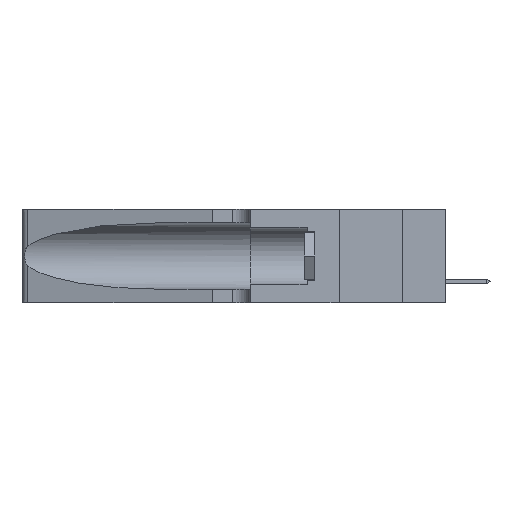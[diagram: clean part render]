
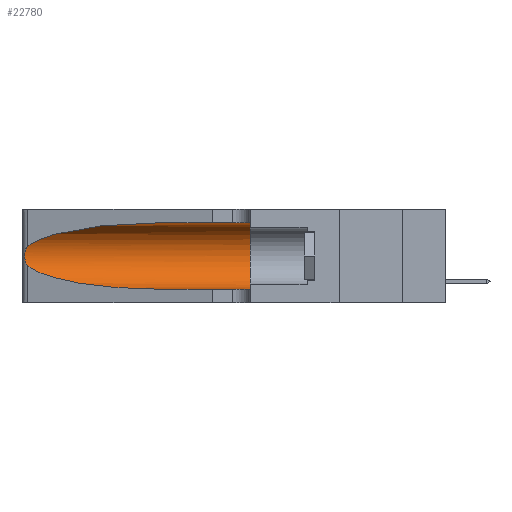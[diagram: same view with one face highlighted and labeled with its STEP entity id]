
A CAD part, left-side view. The second image highlights one B-rep face of the part: STEP entity #22780.
In plain terms, the highlighted cylindrical face has radius 3.308 mm (diameter 6.617 mm), a partial arc.
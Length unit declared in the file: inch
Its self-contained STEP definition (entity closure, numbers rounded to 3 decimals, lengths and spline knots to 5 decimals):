
#247 = ORIENTED_EDGE ( 'NONE', *, *, #14036, .T. ) ;
#489 = EDGE_CURVE ( 'NONE', #13687, #13016, #5493, .T. ) ;
#1385 = CARTESIAN_POINT ( 'NONE',  ( 0.1305, 0.72297, 0.31525 ) ) ;
#1885 = LINE ( 'NONE', #21795, #19134 ) ;
#2237 = CARTESIAN_POINT ( 'NONE',  ( 0.25555, 1.22993, 0.14849 ) ) ;
#2495 = DIRECTION ( 'NONE',  ( 0., -1., 0. ) ) ;
#2584 = CARTESIAN_POINT ( 'NONE',  ( 0.25856, 1.23593, 0.16098 ) ) ;
#2806 = ORIENTED_EDGE ( 'NONE', *, *, #20119, .T. ) ;
#3103 = EDGE_CURVE ( 'NONE', #4375, #17289, #7499, .T. ) ;
#3889 = CARTESIAN_POINT ( 'NONE',  ( 0.25487, 1.22718, 0.14631 ) ) ;
#3930 = CARTESIAN_POINT ( 'NONE',  ( 0.26018, 1.23835, 0.19895 ) ) ;
#4180 =( BOUNDED_CURVE ( )  B_SPLINE_CURVE ( 3, ( #12811, #19799, #11077, #16459 ),
 .UNSPECIFIED., .F., .F. ) 
 B_SPLINE_CURVE_WITH_KNOTS ( ( 4, 4 ),
 ( 3.44316, 4.71239 ),
 .UNSPECIFIED. ) 
 CURVE ( )  GEOMETRIC_REPRESENTATION_ITEM ( )  RATIONAL_B_SPLINE_CURVE ( ( 1., 0.87, 0.87, 1. ) ) 
 REPRESENTATION_ITEM ( '' )  );
#4375 = VERTEX_POINT ( 'NONE', #6279 ) ;
#4800 = CARTESIAN_POINT ( 'NONE',  ( 0.1305, 0.72297, 0.05475 ) ) ;
#5493 = LINE ( 'NONE', #11340, #14532 ) ;
#5975 = CARTESIAN_POINT ( 'NONE',  ( 0.25487, 1.22718, 0.22369 ) ) ;
#6052 = CARTESIAN_POINT ( 'NONE',  ( 0.25487, 1.22718, 0.22369 ) ) ;
#6279 = CARTESIAN_POINT ( 'NONE',  ( 0.25487, 1.22718, 0.22369 ) ) ;
#6394 = CARTESIAN_POINT ( 'NONE',  ( 0.25487, 1.22718, 0.14631 ) ) ;
#7499 = B_SPLINE_CURVE_WITH_KNOTS ( 'NONE', 3,
 ( #6052, #9365, #16404, #11031, #18848, #3930, #15185, #12520, #10865, #2584, #13472, #18225, #2237, #3889 ),
 .UNSPECIFIED., .F., .F.,
 ( 4, 2, 2, 2, 2, 2, 4 ),
 ( 0., 0.00027, 0.00053, 0.00107, 0.0016, 0.00187, 0.00214 ),
 .UNSPECIFIED. ) ;
#7904 = ORIENTED_EDGE ( 'NONE', *, *, #22402, .F. ) ;
#8198 = VERTEX_POINT ( 'NONE', #23181 ) ;
#8211 = EDGE_LOOP ( 'NONE', ( #247, #16313, #2806, #16120, #18876, #7904 ) ) ;
#8506 = CARTESIAN_POINT ( 'NONE',  ( 0.1305, 0.35, 0.185 ) ) ;
#8669 = AXIS2_PLACEMENT_3D ( 'NONE', #8710, #14234, #19709 ) ;
#8710 = CARTESIAN_POINT ( 'NONE',  ( 0.1305, 1.61858, 0.185 ) ) ;
#9045 = CYLINDRICAL_SURFACE ( 'NONE', #8669, 0.13025 ) ;
#9365 = CARTESIAN_POINT ( 'NONE',  ( 0.25555, 1.22994, 0.2215 ) ) ;
#10865 = CARTESIAN_POINT ( 'NONE',  ( 0.26017, 1.23833, 0.17102 ) ) ;
#11031 = CARTESIAN_POINT ( 'NONE',  ( 0.25787, 1.23484, 0.2124 ) ) ;
#11077 = CARTESIAN_POINT ( 'NONE',  ( 0.18966, 0.96281, 0.05475 ) ) ;
#11340 = CARTESIAN_POINT ( 'NONE',  ( 0.1305, 1.61858, 0.05475 ) ) ;
#12191 = DIRECTION ( 'NONE',  ( 0., 1., 0. ) ) ;
#12520 = CARTESIAN_POINT ( 'NONE',  ( 0.26075, 1.23896, 0.178 ) ) ;
#12539 = AXIS2_PLACEMENT_3D ( 'NONE', #8506, #12191, #14628 ) ;
#12811 = CARTESIAN_POINT ( 'NONE',  ( 0.25487, 1.22718, 0.14631 ) ) ;
#13005 = CARTESIAN_POINT ( 'NONE',  ( 0.18966, 0.96281, 0.31525 ) ) ;
#13016 = VERTEX_POINT ( 'NONE', #23282 ) ;
#13472 = CARTESIAN_POINT ( 'NONE',  ( 0.25789, 1.23486, 0.15765 ) ) ;
#13683 = CIRCLE ( 'NONE', #12539, 0.13025 ) ;
#13687 = VERTEX_POINT ( 'NONE', #4800 ) ;
#14036 = EDGE_CURVE ( 'NONE', #19925, #4375, #15338, .T. ) ;
#14234 = DIRECTION ( 'NONE',  ( 0., -1., 0. ) ) ;
#14532 = VECTOR ( 'NONE', #2495, 39.37008 ) ;
#14628 = DIRECTION ( 'NONE',  ( 0., 0., 1. ) ) ;
#15058 = EDGE_CURVE ( 'NONE', #8198, #13016, #13683, .T. ) ;
#15185 = CARTESIAN_POINT ( 'NONE',  ( 0.26075, 1.23896, 0.19203 ) ) ;
#15338 =( BOUNDED_CURVE ( )  B_SPLINE_CURVE ( 3, ( #1385, #13005, #16834, #5975 ),
 .UNSPECIFIED., .F., .F. ) 
 B_SPLINE_CURVE_WITH_KNOTS ( ( 4, 4 ),
 ( 1.5708, 2.84003 ),
 .UNSPECIFIED. ) 
 CURVE ( )  GEOMETRIC_REPRESENTATION_ITEM ( )  RATIONAL_B_SPLINE_CURVE ( ( 1., 0.87, 0.87, 1. ) ) 
 REPRESENTATION_ITEM ( '' )  );
#16116 = FACE_OUTER_BOUND ( 'NONE', #8211, .T. ) ;
#16120 = ORIENTED_EDGE ( 'NONE', *, *, #489, .T. ) ;
#16313 = ORIENTED_EDGE ( 'NONE', *, *, #3103, .T. ) ;
#16404 = CARTESIAN_POINT ( 'NONE',  ( 0.25639, 1.23184, 0.21858 ) ) ;
#16459 = CARTESIAN_POINT ( 'NONE',  ( 0.1305, 0.72297, 0.05475 ) ) ;
#16834 = CARTESIAN_POINT ( 'NONE',  ( 0.2373, 1.15595, 0.28018 ) ) ;
#17289 = VERTEX_POINT ( 'NONE', #6394 ) ;
#18225 = CARTESIAN_POINT ( 'NONE',  ( 0.25639, 1.23186, 0.15144 ) ) ;
#18848 = CARTESIAN_POINT ( 'NONE',  ( 0.25854, 1.2359, 0.20912 ) ) ;
#18876 = ORIENTED_EDGE ( 'NONE', *, *, #15058, .F. ) ;
#19134 = VECTOR ( 'NONE', #22038, 39.37008 ) ;
#19709 = DIRECTION ( 'NONE',  ( 0., 0., -1. ) ) ;
#19799 = CARTESIAN_POINT ( 'NONE',  ( 0.2373, 1.15595, 0.08982 ) ) ;
#19925 = VERTEX_POINT ( 'NONE', #20430 ) ;
#20119 = EDGE_CURVE ( 'NONE', #17289, #13687, #4180, .T. ) ;
#20430 = CARTESIAN_POINT ( 'NONE',  ( 0.1305, 0.72297, 0.31525 ) ) ;
#21795 = CARTESIAN_POINT ( 'NONE',  ( 0.1305, 1.61858, 0.31525 ) ) ;
#22038 = DIRECTION ( 'NONE',  ( 0., -1., 0. ) ) ;
#22402 = EDGE_CURVE ( 'NONE', #19925, #8198, #1885, .T. ) ;
#22780 = ADVANCED_FACE ( 'NONE', ( #16116 ), #9045, .F. ) ;
#23181 = CARTESIAN_POINT ( 'NONE',  ( 0.1305, 0.35, 0.31525 ) ) ;
#23282 = CARTESIAN_POINT ( 'NONE',  ( 0.1305, 0.35, 0.05475 ) ) ;
